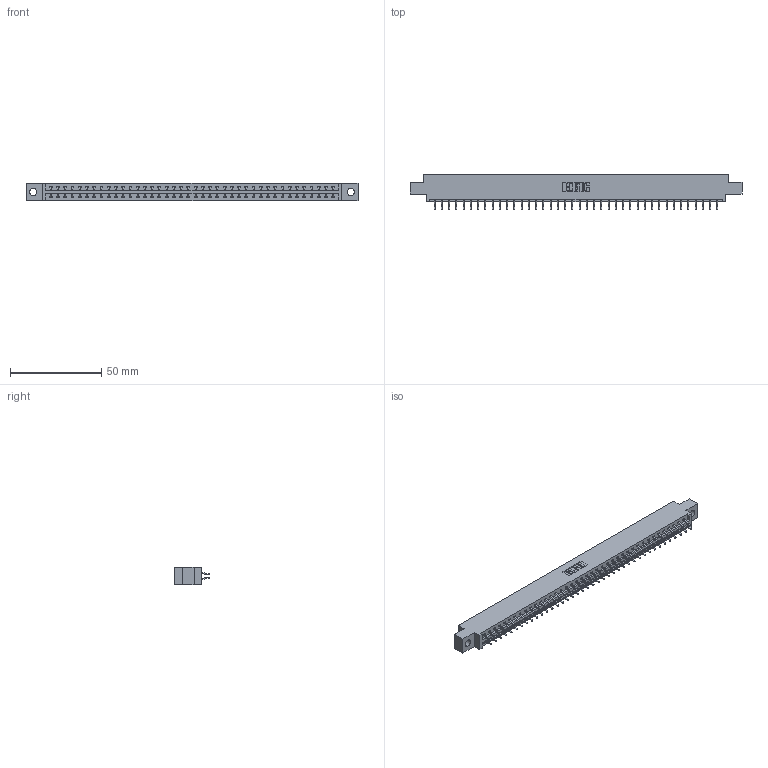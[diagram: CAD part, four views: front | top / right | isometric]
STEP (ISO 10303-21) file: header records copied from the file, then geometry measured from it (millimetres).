
FILE_DESCRIPTION (( 'STEP AP203' ), '1' );
FILE_NAME ('337-080-556-804.STEP', '2018-08-12T18:46:43', ( '' ), ( '' ), 'SwSTEP 2.0', 'SolidWorks 2016', '' );
FILE_SCHEMA (( 'CONFIG_CONTROL_DESIGN' ));
Length unit declared in the file: inch
Products named in the file (3): 337 Part_0.170 Offset - 0.156 Dia-TH; 345-292-001_556 Tail; 337-080-556-804
Assembly tree (81 placements, depth 2):
  337-080-556-804
    337 Part_0.170 Offset - 0.156 Dia-TH
    345-292-001_556 Tail  x80
Bounding box: 181.51 x 19.57 x 9.4 mm (x, y, z)
Volume: 18893.6 mm3; surface area: 21160.7 mm2
Topology: 81 solids, 81 shells, 4918 faces, 14643 edges, 9654 vertices
Faces by surface type: plane 3434, cylinder 1484
Entity records: 31627 total; most frequent: CARTESIAN_POINT 5346, ORIENTED_EDGE 5270, DIRECTION 4539, EDGE_CURVE 2635, VECTOR 2499, LINE 2499, VERTEX_POINT 1754, AXIS2_PLACEMENT_3D 1020
